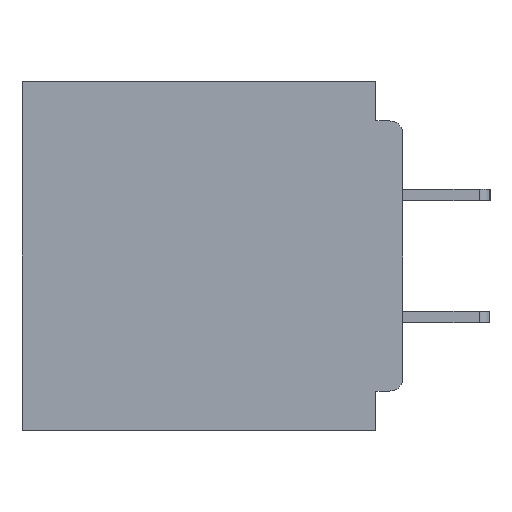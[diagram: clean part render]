
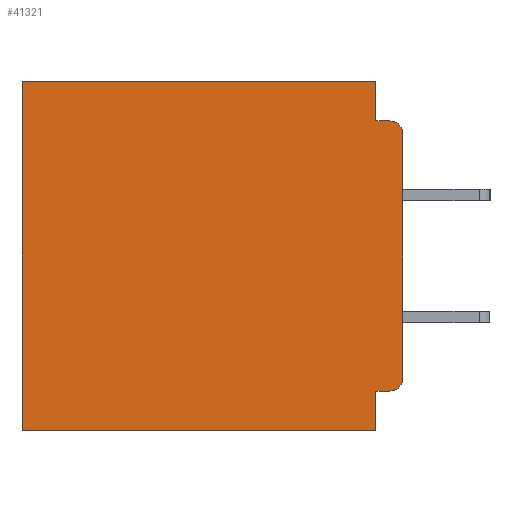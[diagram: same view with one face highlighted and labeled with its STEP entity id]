
A CAD part, left-side view. The second image highlights one B-rep face of the part: STEP entity #41321.
In plain terms, the highlighted planar face has unit normal (-1, 0, 0).
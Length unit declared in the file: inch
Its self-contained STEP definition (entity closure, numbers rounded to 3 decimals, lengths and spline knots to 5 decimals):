
#46 = CIRCLE ( 'NONE', #41300, 0.015 ) ;
#607 = LINE ( 'NONE', #1154, #25608 ) ;
#797 = VERTEX_POINT ( 'NONE', #40420 ) ;
#856 = LINE ( 'NONE', #11604, #33327 ) ;
#1128 = CARTESIAN_POINT ( 'NONE',  ( 0.3, 0.015, -0.06 ) ) ;
#1138 = ORIENTED_EDGE ( 'NONE', *, *, #35712, .F. ) ;
#1154 = CARTESIAN_POINT ( 'NONE',  ( 0.3, 0., -0.4 ) ) ;
#1873 = ORIENTED_EDGE ( 'NONE', *, *, #8532, .F. ) ;
#2513 = VERTEX_POINT ( 'NONE', #8434 ) ;
#2884 = ORIENTED_EDGE ( 'NONE', *, *, #6498, .T. ) ;
#3091 = VECTOR ( 'NONE', #11715, 39.37008 ) ;
#3155 = CARTESIAN_POINT ( 'NONE',  ( 0.3, 0.015, -0.34 ) ) ;
#3757 = EDGE_CURVE ( 'NONE', #39255, #36920, #856, .T. ) ;
#3814 = EDGE_CURVE ( 'NONE', #13515, #16416, #6483, .T. ) ;
#4421 = DIRECTION ( 'NONE',  ( 0., 0., -1. ) ) ;
#4534 = CARTESIAN_POINT ( 'NONE',  ( 0.3, 0., 0. ) ) ;
#5071 = DIRECTION ( 'NONE',  ( 0., 1., 0. ) ) ;
#5266 = AXIS2_PLACEMENT_3D ( 'NONE', #17369, #39925, #20643 ) ;
#6436 = DIRECTION ( 'NONE',  ( 0., 0., -1. ) ) ;
#6483 = LINE ( 'NONE', #4534, #22797 ) ;
#6498 = EDGE_CURVE ( 'NONE', #16416, #34606, #12733, .T. ) ;
#8277 = ORIENTED_EDGE ( 'NONE', *, *, #9000, .T. ) ;
#8434 = CARTESIAN_POINT ( 'NONE',  ( 0.3, 0.015, -0.045 ) ) ;
#8532 = EDGE_CURVE ( 'NONE', #14872, #34606, #18654, .T. ) ;
#8780 = CARTESIAN_POINT ( 'NONE',  ( 0.3, 0.437, -0.4 ) ) ;
#9000 = EDGE_CURVE ( 'NONE', #797, #2513, #36793, .T. ) ;
#9830 = CARTESIAN_POINT ( 'NONE',  ( 0.3, 0.031, -0.4 ) ) ;
#9961 = ORIENTED_EDGE ( 'NONE', *, *, #3814, .T. ) ;
#10013 = VECTOR ( 'NONE', #40772, 39.37008 ) ;
#10797 = CARTESIAN_POINT ( 'NONE',  ( 0.3, 0.031, -0.045 ) ) ;
#11066 = CARTESIAN_POINT ( 'NONE',  ( 0.3, 0.031, 0. ) ) ;
#11604 = CARTESIAN_POINT ( 'NONE',  ( 0.3, 0., -0.355 ) ) ;
#11715 = DIRECTION ( 'NONE',  ( 0., 0., -1. ) ) ;
#11907 = CARTESIAN_POINT ( 'NONE',  ( 0.3, 0.437, -0.4 ) ) ;
#11921 = CARTESIAN_POINT ( 'NONE',  ( 0.3, 0.437, 0. ) ) ;
#12301 = CARTESIAN_POINT ( 'NONE',  ( 0.3, 0.031, -0.355 ) ) ;
#12733 = LINE ( 'NONE', #11907, #3091 ) ;
#13017 = LINE ( 'NONE', #40411, #35789 ) ;
#13281 = EDGE_CURVE ( 'NONE', #36920, #14872, #37070, .T. ) ;
#13515 = VERTEX_POINT ( 'NONE', #11066 ) ;
#14087 = PLANE ( 'NONE',  #5266 ) ;
#14869 = AXIS2_PLACEMENT_3D ( 'NONE', #1128, #23957, #4421 ) ;
#14872 = VERTEX_POINT ( 'NONE', #27924 ) ;
#15194 = VERTEX_POINT ( 'NONE', #10797 ) ;
#16124 = LINE ( 'NONE', #18602, #23825 ) ;
#16416 = VERTEX_POINT ( 'NONE', #11921 ) ;
#17369 = CARTESIAN_POINT ( 'NONE',  ( 0.3, 0., -0.4 ) ) ;
#18602 = CARTESIAN_POINT ( 'NONE',  ( 0.3, 0., -0.045 ) ) ;
#18654 = LINE ( 'NONE', #21528, #10013 ) ;
#19019 = ORIENTED_EDGE ( 'NONE', *, *, #29590, .F. ) ;
#19813 = CARTESIAN_POINT ( 'NONE',  ( 0.3, 0.015, -0.355 ) ) ;
#20636 = DIRECTION ( 'NONE',  ( 0., 0., -1. ) ) ;
#20643 = DIRECTION ( 'NONE',  ( 0., 0., -1. ) ) ;
#21528 = CARTESIAN_POINT ( 'NONE',  ( 0.3, 0., -0.4 ) ) ;
#22453 = DIRECTION ( 'NONE',  ( 0., 1., 0. ) ) ;
#22797 = VECTOR ( 'NONE', #5071, 39.37008 ) ;
#23616 = FACE_OUTER_BOUND ( 'NONE', #36349, .T. ) ;
#23637 = EDGE_CURVE ( 'NONE', #13515, #15194, #13017, .T. ) ;
#23825 = VECTOR ( 'NONE', #34683, 39.37008 ) ;
#23845 = ORIENTED_EDGE ( 'NONE', *, *, #3757, .F. ) ;
#23957 = DIRECTION ( 'NONE',  ( -1., 0., 0. ) ) ;
#25608 = VECTOR ( 'NONE', #20636, 39.37008 ) ;
#25958 = DIRECTION ( 'NONE',  ( -1., 0., 0. ) ) ;
#26787 = ORIENTED_EDGE ( 'NONE', *, *, #23637, .F. ) ;
#27924 = CARTESIAN_POINT ( 'NONE',  ( 0.3, 0.031, -0.4 ) ) ;
#28624 = VECTOR ( 'NONE', #32487, 39.37008 ) ;
#29590 = EDGE_CURVE ( 'NONE', #15194, #2513, #16124, .T. ) ;
#32487 = DIRECTION ( 'NONE',  ( 0., 0., -1. ) ) ;
#33327 = VECTOR ( 'NONE', #22453, 39.37008 ) ;
#34606 = VERTEX_POINT ( 'NONE', #8780 ) ;
#34683 = DIRECTION ( 'NONE',  ( 0., -1., 0. ) ) ;
#35712 = EDGE_CURVE ( 'NONE', #797, #37508, #607, .T. ) ;
#35789 = VECTOR ( 'NONE', #37328, 39.37008 ) ;
#36349 = EDGE_LOOP ( 'NONE', ( #1138, #8277, #19019, #26787, #9961, #2884, #1873, #36369, #23845, #37408 ) ) ;
#36369 = ORIENTED_EDGE ( 'NONE', *, *, #13281, .F. ) ;
#36793 = CIRCLE ( 'NONE', #14869, 0.015 ) ;
#36920 = VERTEX_POINT ( 'NONE', #12301 ) ;
#37070 = LINE ( 'NONE', #9830, #28624 ) ;
#37328 = DIRECTION ( 'NONE',  ( 0., 0., -1. ) ) ;
#37408 = ORIENTED_EDGE ( 'NONE', *, *, #41922, .T. ) ;
#37508 = VERTEX_POINT ( 'NONE', #41036 ) ;
#39255 = VERTEX_POINT ( 'NONE', #19813 ) ;
#39925 = DIRECTION ( 'NONE',  ( 1., 0., 0. ) ) ;
#40411 = CARTESIAN_POINT ( 'NONE',  ( 0.3, 0.031, 0. ) ) ;
#40420 = CARTESIAN_POINT ( 'NONE',  ( 0.3, 0., -0.06 ) ) ;
#40772 = DIRECTION ( 'NONE',  ( 0., 1., 0. ) ) ;
#41036 = CARTESIAN_POINT ( 'NONE',  ( 0.3, 0., -0.34 ) ) ;
#41300 = AXIS2_PLACEMENT_3D ( 'NONE', #3155, #25958, #6436 ) ;
#41321 = ADVANCED_FACE ( 'NONE', ( #23616 ), #14087, .F. ) ;
#41922 = EDGE_CURVE ( 'NONE', #39255, #37508, #46, .T. ) ;
